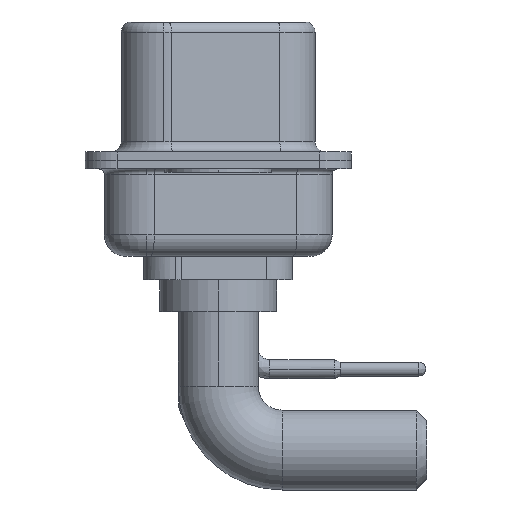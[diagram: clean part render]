
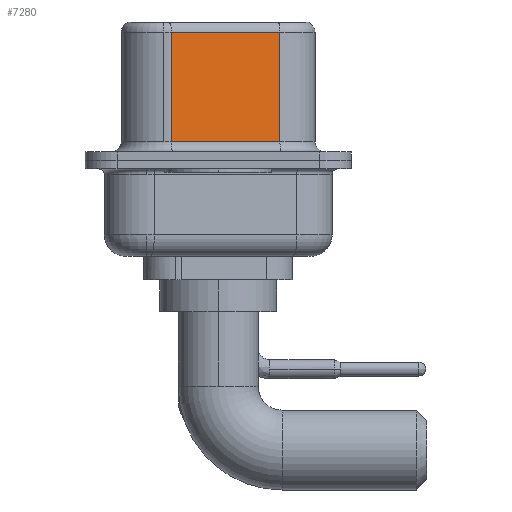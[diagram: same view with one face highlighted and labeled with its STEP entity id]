
A CAD part, left-side view. The second image highlights one B-rep face of the part: STEP entity #7280.
In plain terms, the highlighted planar face has unit normal (-0.985, -0.174, 0).
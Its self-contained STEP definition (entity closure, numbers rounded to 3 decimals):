
#1139 = EDGE_CURVE ( 'NONE', #15238, #16557, #10426, .T. ) ;
#2070 = ORIENTED_EDGE ( 'NONE', *, *, #20958, .T. ) ;
#2532 = ORIENTED_EDGE ( 'NONE', *, *, #19254, .F. ) ;
#3118 = DIRECTION ( 'NONE',  ( 0.985, 0.174, 0. ) ) ;
#4171 = CARTESIAN_POINT ( 'NONE',  ( 4.58, -2.897, 6.02 ) ) ;
#4309 = VECTOR ( 'NONE', #15989, 1000. ) ;
#4449 = VERTEX_POINT ( 'NONE', #15039 ) ;
#4924 = LINE ( 'NONE', #11994, #21448 ) ;
#5184 = LINE ( 'NONE', #6808, #22549 ) ;
#6808 = CARTESIAN_POINT ( 'NONE',  ( 4.58, -2.897, 6.52 ) ) ;
#7280 = ADVANCED_FACE ( 'NONE', ( #9322 ), #8699, .F. ) ;
#7314 = LINE ( 'NONE', #4171, #16604 ) ;
#8286 = EDGE_CURVE ( 'NONE', #4449, #19482, #7314, .T. ) ;
#8699 = PLANE ( 'NONE',  #16196 ) ;
#9322 = FACE_OUTER_BOUND ( 'NONE', #10182, .T. ) ;
#9392 = CARTESIAN_POINT ( 'NONE',  ( 3.68, 2.203, 0.9 ) ) ;
#10182 = EDGE_LOOP ( 'NONE', ( #2532, #21087, #2070, #12281 ) ) ;
#10426 = LINE ( 'NONE', #12395, #4309 ) ;
#10613 = DIRECTION ( 'NONE',  ( 0., 0., -1. ) ) ;
#11994 = CARTESIAN_POINT ( 'NONE',  ( 3.68, 2.203, 6.52 ) ) ;
#12281 = ORIENTED_EDGE ( 'NONE', *, *, #1139, .T. ) ;
#12285 = CARTESIAN_POINT ( 'NONE',  ( 4.58, -2.897, 6.52 ) ) ;
#12395 = CARTESIAN_POINT ( 'NONE',  ( 4.58, -2.897, 0.9 ) ) ;
#12758 = CARTESIAN_POINT ( 'NONE',  ( 4.58, -2.897, 0.9 ) ) ;
#15039 = CARTESIAN_POINT ( 'NONE',  ( 4.58, -2.897, 6.02 ) ) ;
#15238 = VERTEX_POINT ( 'NONE', #9392 ) ;
#15751 = DIRECTION ( 'NONE',  ( -0.174, 0.985, 0. ) ) ;
#15989 = DIRECTION ( 'NONE',  ( 0.174, -0.985, 0. ) ) ;
#16196 = AXIS2_PLACEMENT_3D ( 'NONE', #12285, #3118, #15751 ) ;
#16557 = VERTEX_POINT ( 'NONE', #12758 ) ;
#16604 = VECTOR ( 'NONE', #21475, 1000. ) ;
#19072 = DIRECTION ( 'NONE',  ( 0., 0., -1. ) ) ;
#19254 = EDGE_CURVE ( 'NONE', #4449, #16557, #5184, .T. ) ;
#19482 = VERTEX_POINT ( 'NONE', #22428 ) ;
#20958 = EDGE_CURVE ( 'NONE', #19482, #15238, #4924, .T. ) ;
#21087 = ORIENTED_EDGE ( 'NONE', *, *, #8286, .T. ) ;
#21448 = VECTOR ( 'NONE', #19072, 1000. ) ;
#21475 = DIRECTION ( 'NONE',  ( -0.174, 0.985, 0. ) ) ;
#22428 = CARTESIAN_POINT ( 'NONE',  ( 3.68, 2.203, 6.02 ) ) ;
#22549 = VECTOR ( 'NONE', #10613, 1000. ) ;
